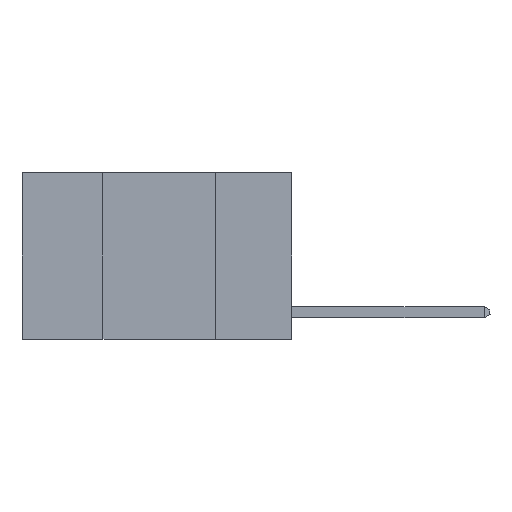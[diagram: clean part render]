
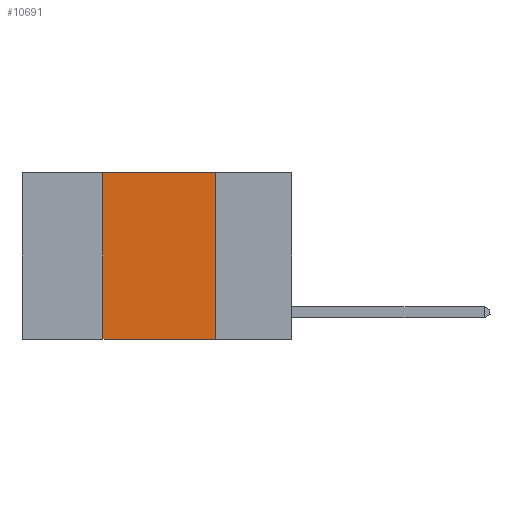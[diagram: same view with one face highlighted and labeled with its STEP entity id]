
A CAD part, left-side view. The second image highlights one B-rep face of the part: STEP entity #10691.
In plain terms, the highlighted planar face has unit normal (-1, 0, 0).
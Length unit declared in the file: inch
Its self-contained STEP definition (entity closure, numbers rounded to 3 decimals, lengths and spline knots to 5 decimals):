
#44 = DIRECTION ( 'NONE',  ( 1., 0., 0. ) ) ;
#4495 = ORIENTED_EDGE ( 'NONE', *, *, #12608, .F. ) ;
#4729 = CARTESIAN_POINT ( 'NONE',  ( 0., 0.17, 0. ) ) ;
#5955 = LINE ( 'NONE', #20904, #8416 ) ;
#5972 = CARTESIAN_POINT ( 'NONE',  ( 0., 0.17, 0. ) ) ;
#6068 = DIRECTION ( 'NONE',  ( 0., -1., 0. ) ) ;
#6578 = EDGE_CURVE ( 'NONE', #15594, #15539, #23437, .T. ) ;
#8416 = VECTOR ( 'NONE', #6068, 39.37008 ) ;
#8629 = DIRECTION ( 'NONE',  ( 0., 0., -1. ) ) ;
#8722 = ORIENTED_EDGE ( 'NONE', *, *, #6578, .F. ) ;
#9622 = ORIENTED_EDGE ( 'NONE', *, *, #15460, .T. ) ;
#10691 = ADVANCED_FACE ( 'NONE', ( #12898 ), #20362, .F. ) ;
#11237 = CARTESIAN_POINT ( 'NONE',  ( 0., 0.42, 0. ) ) ;
#12608 = EDGE_CURVE ( 'NONE', #22020, #19661, #16681, .T. ) ;
#12667 = VECTOR ( 'NONE', #14695, 39.37008 ) ;
#12898 = FACE_OUTER_BOUND ( 'NONE', #23940, .T. ) ;
#14578 = LINE ( 'NONE', #22128, #12667 ) ;
#14695 = DIRECTION ( 'NONE',  ( 0., -1., 0. ) ) ;
#14963 = EDGE_CURVE ( 'NONE', #19661, #15594, #5955, .T. ) ;
#15460 = EDGE_CURVE ( 'NONE', #22020, #15539, #14578, .T. ) ;
#15539 = VERTEX_POINT ( 'NONE', #20706 ) ;
#15594 = VERTEX_POINT ( 'NONE', #5972 ) ;
#15835 = AXIS2_PLACEMENT_3D ( 'NONE', #16673, #44, #22284 ) ;
#16673 = CARTESIAN_POINT ( 'NONE',  ( 0., 0.6, 0. ) ) ;
#16681 = LINE ( 'NONE', #11237, #16768 ) ;
#16768 = VECTOR ( 'NONE', #20619, 39.37008 ) ;
#16992 = CARTESIAN_POINT ( 'NONE',  ( 0., 0.42, 0. ) ) ;
#17400 = CARTESIAN_POINT ( 'NONE',  ( 0., 0.42, -0.37 ) ) ;
#17526 = ORIENTED_EDGE ( 'NONE', *, *, #14963, .F. ) ;
#19164 = VECTOR ( 'NONE', #8629, 39.37008 ) ;
#19661 = VERTEX_POINT ( 'NONE', #16992 ) ;
#20362 = PLANE ( 'NONE',  #15835 ) ;
#20619 = DIRECTION ( 'NONE',  ( 0., 0., 1. ) ) ;
#20706 = CARTESIAN_POINT ( 'NONE',  ( 0., 0.17, -0.37 ) ) ;
#20904 = CARTESIAN_POINT ( 'NONE',  ( 0., 0.6, 0. ) ) ;
#22020 = VERTEX_POINT ( 'NONE', #17400 ) ;
#22128 = CARTESIAN_POINT ( 'NONE',  ( 0., 0.6, -0.37 ) ) ;
#22284 = DIRECTION ( 'NONE',  ( 0., 0., -1. ) ) ;
#23437 = LINE ( 'NONE', #4729, #19164 ) ;
#23940 = EDGE_LOOP ( 'NONE', ( #8722, #17526, #4495, #9622 ) ) ;
